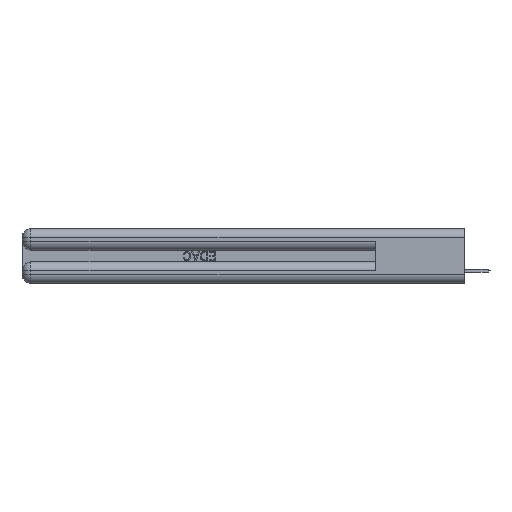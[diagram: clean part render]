
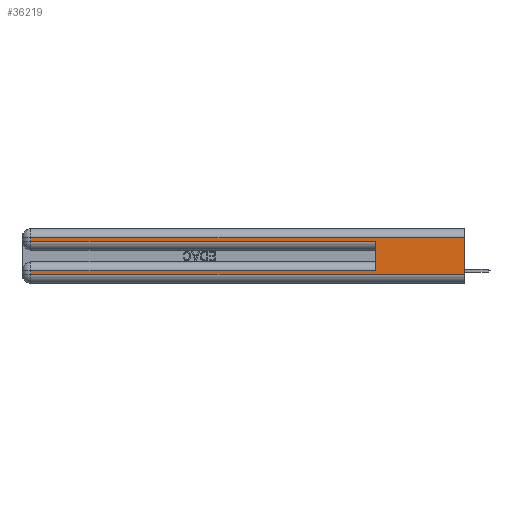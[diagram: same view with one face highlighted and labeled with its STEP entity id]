
A CAD part, left-side view. The second image highlights one B-rep face of the part: STEP entity #36219.
In plain terms, the highlighted planar face has unit normal (-1, 0, 0).
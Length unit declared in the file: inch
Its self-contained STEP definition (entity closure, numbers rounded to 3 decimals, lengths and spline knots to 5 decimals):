
#1477 = DIRECTION ( 'NONE',  ( 0., 1., 0. ) ) ;
#2235 = CARTESIAN_POINT ( 'NONE',  ( 0., 0., 0.285 ) ) ;
#2437 = VERTEX_POINT ( 'NONE', #29849 ) ;
#2775 = ORIENTED_EDGE ( 'NONE', *, *, #18828, .F. ) ;
#2841 = EDGE_CURVE ( 'NONE', #40210, #42033, #25230, .T. ) ;
#4413 = CARTESIAN_POINT ( 'NONE',  ( 0., 0., 0.37 ) ) ;
#4728 = CARTESIAN_POINT ( 'NONE',  ( 0., 0., 0.31 ) ) ;
#6410 = LINE ( 'NONE', #2235, #44023 ) ;
#6543 = DIRECTION ( 'NONE',  ( 0., 0., -1. ) ) ;
#6835 = DIRECTION ( 'NONE',  ( 0., 0., -1. ) ) ;
#8230 = LINE ( 'NONE', #9670, #17051 ) ;
#8335 = DIRECTION ( 'NONE',  ( 0., 0., -1. ) ) ;
#9670 = CARTESIAN_POINT ( 'NONE',  ( 0., 0., 0.085 ) ) ;
#10032 = ORIENTED_EDGE ( 'NONE', *, *, #12707, .T. ) ;
#11904 = LINE ( 'NONE', #42835, #37267 ) ;
#12017 = CARTESIAN_POINT ( 'NONE',  ( 0., 0.6, 0.285 ) ) ;
#12280 = EDGE_CURVE ( 'NONE', #22366, #42033, #40601, .T. ) ;
#12707 = EDGE_CURVE ( 'NONE', #45941, #21647, #6410, .T. ) ;
#13375 = CARTESIAN_POINT ( 'NONE',  ( 0., 0., 0.06 ) ) ;
#15209 = VECTOR ( 'NONE', #6835, 39.37008 ) ;
#15851 = CARTESIAN_POINT ( 'NONE',  ( 0., 2.94, 0.085 ) ) ;
#16818 = CARTESIAN_POINT ( 'NONE',  ( 0., 2.94, 0.06 ) ) ;
#17051 = VECTOR ( 'NONE', #20793, 39.37008 ) ;
#17056 = CARTESIAN_POINT ( 'NONE',  ( 0., 2.94, 0.285 ) ) ;
#18828 = EDGE_CURVE ( 'NONE', #2437, #21647, #11904, .T. ) ;
#19811 = EDGE_CURVE ( 'NONE', #44670, #22366, #40707, .T. ) ;
#19962 = EDGE_CURVE ( 'NONE', #2437, #44670, #8230, .T. ) ;
#20793 = DIRECTION ( 'NONE',  ( 0., 1., 0. ) ) ;
#21647 = VERTEX_POINT ( 'NONE', #12017 ) ;
#22366 = VERTEX_POINT ( 'NONE', #16818 ) ;
#22965 = EDGE_CURVE ( 'NONE', #46899, #45941, #26838, .T. ) ;
#23101 = FACE_OUTER_BOUND ( 'NONE', #34095, .T. ) ;
#24064 = DIRECTION ( 'NONE',  ( 0., 0., 1. ) ) ;
#24955 = PLANE ( 'NONE',  #46694 ) ;
#25230 = LINE ( 'NONE', #4413, #15209 ) ;
#26037 = CARTESIAN_POINT ( 'NONE',  ( 0., 2.94, 0.31 ) ) ;
#26838 = LINE ( 'NONE', #31061, #40989 ) ;
#28937 = CARTESIAN_POINT ( 'NONE',  ( 0., 0., 0.06 ) ) ;
#29095 = DIRECTION ( 'NONE',  ( 1., 0., 0. ) ) ;
#29418 = ORIENTED_EDGE ( 'NONE', *, *, #2841, .F. ) ;
#29849 = CARTESIAN_POINT ( 'NONE',  ( 0., 0.6, 0.085 ) ) ;
#30633 = VECTOR ( 'NONE', #8335, 39.37008 ) ;
#31061 = CARTESIAN_POINT ( 'NONE',  ( 0., 2.94, 0.37 ) ) ;
#31346 = CARTESIAN_POINT ( 'NONE',  ( 0., 2.94, 0.37 ) ) ;
#32070 = VECTOR ( 'NONE', #1477, 39.37008 ) ;
#32535 = CARTESIAN_POINT ( 'NONE',  ( 0., 0., 0.37 ) ) ;
#32608 = ORIENTED_EDGE ( 'NONE', *, *, #19811, .T. ) ;
#32614 = DIRECTION ( 'NONE',  ( 0., -1., 0. ) ) ;
#32687 = ORIENTED_EDGE ( 'NONE', *, *, #22965, .T. ) ;
#34095 = EDGE_LOOP ( 'NONE', ( #29418, #42885, #32687, #10032, #2775, #43388, #32608, #35204 ) ) ;
#35204 = ORIENTED_EDGE ( 'NONE', *, *, #12280, .T. ) ;
#35887 = CARTESIAN_POINT ( 'NONE',  ( 0., 0., 0.31 ) ) ;
#36219 = ADVANCED_FACE ( 'NONE', ( #23101 ), #24955, .F. ) ;
#37078 = VECTOR ( 'NONE', #32614, 39.37008 ) ;
#37267 = VECTOR ( 'NONE', #24064, 39.37008 ) ;
#38345 = DIRECTION ( 'NONE',  ( 0., 0., -1. ) ) ;
#39176 = LINE ( 'NONE', #35887, #32070 ) ;
#40210 = VERTEX_POINT ( 'NONE', #4728 ) ;
#40601 = LINE ( 'NONE', #13375, #37078 ) ;
#40707 = LINE ( 'NONE', #31346, #30633 ) ;
#40989 = VECTOR ( 'NONE', #38345, 39.37008 ) ;
#42033 = VERTEX_POINT ( 'NONE', #28937 ) ;
#42835 = CARTESIAN_POINT ( 'NONE',  ( 0., 0.6, 0.145 ) ) ;
#42885 = ORIENTED_EDGE ( 'NONE', *, *, #48247, .T. ) ;
#43388 = ORIENTED_EDGE ( 'NONE', *, *, #19962, .T. ) ;
#44023 = VECTOR ( 'NONE', #47402, 39.37008 ) ;
#44670 = VERTEX_POINT ( 'NONE', #15851 ) ;
#45941 = VERTEX_POINT ( 'NONE', #17056 ) ;
#46694 = AXIS2_PLACEMENT_3D ( 'NONE', #32535, #29095, #6543 ) ;
#46899 = VERTEX_POINT ( 'NONE', #26037 ) ;
#47402 = DIRECTION ( 'NONE',  ( 0., -1., 0. ) ) ;
#48247 = EDGE_CURVE ( 'NONE', #40210, #46899, #39176, .T. ) ;
